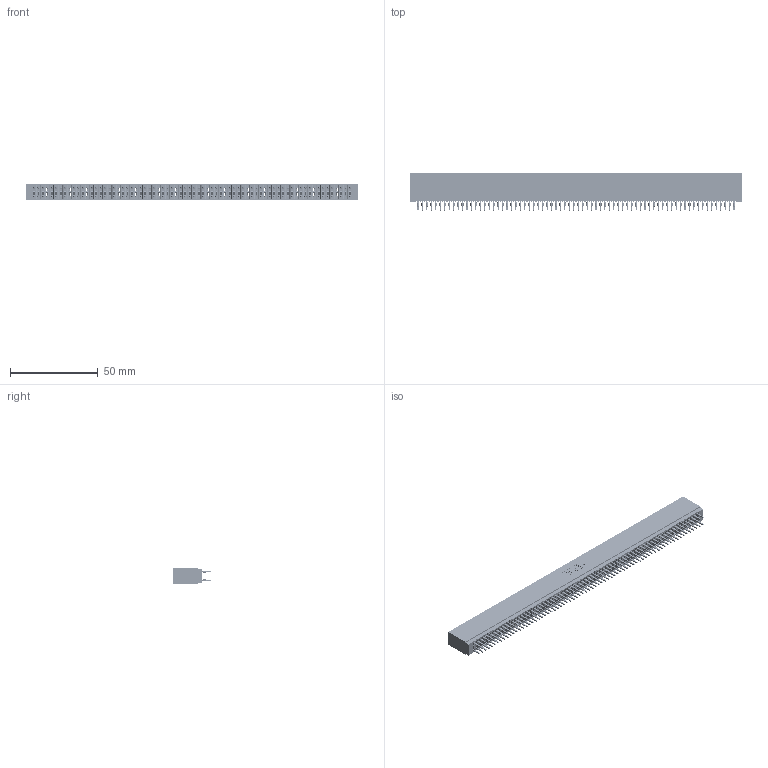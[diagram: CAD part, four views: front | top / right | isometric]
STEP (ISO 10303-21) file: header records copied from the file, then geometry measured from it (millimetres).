
FILE_DESCRIPTION (( 'STEP AP203' ), '1' );
FILE_NAME ('745-144-560-201.STEP', '2026-02-27T04:23:36', ( '' ), ( '' ), 'SwSTEP 2.0', 'SolidWorks 2023', '' );
FILE_SCHEMA (( 'CONFIG_CONTROL_DESIGN' ));
Length unit declared in the file: millimetre
Products named in the file (3): 745-292-001_560; 745 Part_Insulator Option - 01; 745-144-560-201
Assembly tree (145 placements, depth 2):
  745-144-560-201
    745 Part_Insulator Option - 01
    745-292-001_560  x144
Bounding box: 189.48 x 21.22 x 8.89 mm (x, y, z)
Volume: 17416.1 mm3; surface area: 38371.1 mm2
Topology: 145 solids, 145 shells, 14279 faces, 39066 edges, 24796 vertices
Faces by surface type: plane 7399, cylinder 3136, bspline 2880, torus 864
Entity records: 117441 total; most frequent: CARTESIAN_POINT 20865, ORIENTED_EDGE 20360, DIRECTION 17764, EDGE_CURVE 10180, LINE 9558, VECTOR 9558, VERTEX_POINT 6492, AXIS2_PLACEMENT_3D 4103
